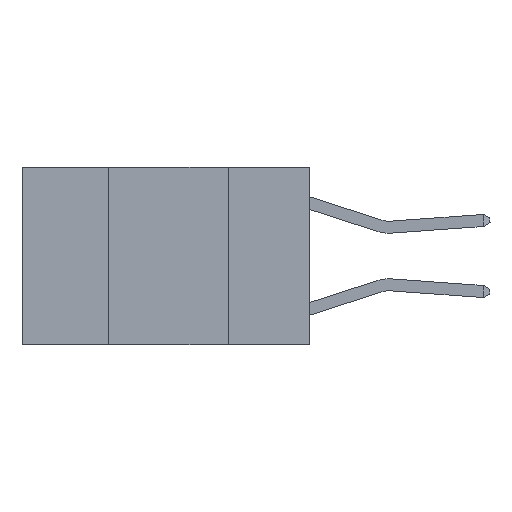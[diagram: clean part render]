
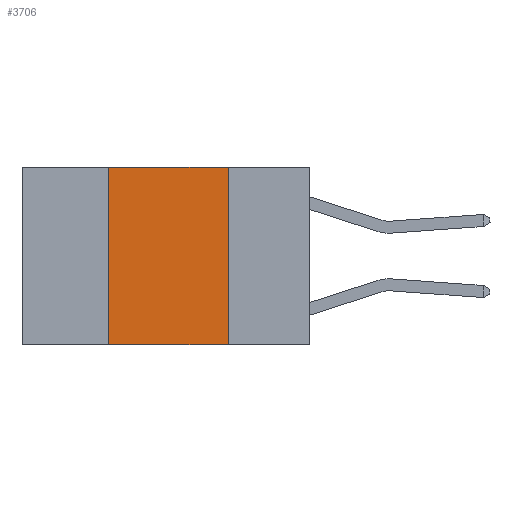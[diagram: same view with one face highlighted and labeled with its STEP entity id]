
A CAD part, left-side view. The second image highlights one B-rep face of the part: STEP entity #3706.
In plain terms, the highlighted planar face has unit normal (-1, 0, 0).
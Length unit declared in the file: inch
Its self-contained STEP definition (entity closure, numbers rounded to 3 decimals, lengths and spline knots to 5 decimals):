
#1372 = PLANE ( 'NONE',  #6216 ) ;
#1774 = EDGE_CURVE ( 'NONE', #10091, #12198, #4203, .T. ) ;
#2193 = ORIENTED_EDGE ( 'NONE', *, *, #7167, .F. ) ;
#2509 = VERTEX_POINT ( 'NONE', #12847 ) ;
#2568 = CARTESIAN_POINT ( 'NONE',  ( 0., 0.6, 0. ) ) ;
#2668 = EDGE_LOOP ( 'NONE', ( #5587, #2193, #8584, #11787 ) ) ;
#3404 = VECTOR ( 'NONE', #7515, 39.37008 ) ;
#3407 = DIRECTION ( 'NONE',  ( 0., 0., -1. ) ) ;
#3453 = EDGE_CURVE ( 'NONE', #2509, #6260, #5759, .T. ) ;
#3706 = ADVANCED_FACE ( 'NONE', ( #4728 ), #1372, .F. ) ;
#3886 = DIRECTION ( 'NONE',  ( 1., 0., 0. ) ) ;
#4203 = LINE ( 'NONE', #15080, #3404 ) ;
#4728 = FACE_OUTER_BOUND ( 'NONE', #2668, .T. ) ;
#5340 = VECTOR ( 'NONE', #3407, 39.37008 ) ;
#5442 = VECTOR ( 'NONE', #14764, 39.37008 ) ;
#5587 = ORIENTED_EDGE ( 'NONE', *, *, #3453, .F. ) ;
#5759 = LINE ( 'NONE', #13618, #5340 ) ;
#6216 = AXIS2_PLACEMENT_3D ( 'NONE', #2568, #3886, #12817 ) ;
#6260 = VERTEX_POINT ( 'NONE', #14346 ) ;
#6688 = LINE ( 'NONE', #9633, #10096 ) ;
#7045 = DIRECTION ( 'NONE',  ( 0., -1., 0. ) ) ;
#7167 = EDGE_CURVE ( 'NONE', #12198, #2509, #12240, .T. ) ;
#7515 = DIRECTION ( 'NONE',  ( 0., 0., 1. ) ) ;
#8584 = ORIENTED_EDGE ( 'NONE', *, *, #1774, .F. ) ;
#9633 = CARTESIAN_POINT ( 'NONE',  ( 0., 0.6, -0.37 ) ) ;
#10091 = VERTEX_POINT ( 'NONE', #12140 ) ;
#10096 = VECTOR ( 'NONE', #7045, 39.37008 ) ;
#11787 = ORIENTED_EDGE ( 'NONE', *, *, #14855, .T. ) ;
#12140 = CARTESIAN_POINT ( 'NONE',  ( 0., 0.42, -0.37 ) ) ;
#12198 = VERTEX_POINT ( 'NONE', #14069 ) ;
#12240 = LINE ( 'NONE', #15957, #5442 ) ;
#12817 = DIRECTION ( 'NONE',  ( 0., 0., -1. ) ) ;
#12847 = CARTESIAN_POINT ( 'NONE',  ( 0., 0.17, 0. ) ) ;
#13618 = CARTESIAN_POINT ( 'NONE',  ( 0., 0.17, 0. ) ) ;
#14069 = CARTESIAN_POINT ( 'NONE',  ( 0., 0.42, 0. ) ) ;
#14346 = CARTESIAN_POINT ( 'NONE',  ( 0., 0.17, -0.37 ) ) ;
#14764 = DIRECTION ( 'NONE',  ( 0., -1., 0. ) ) ;
#14855 = EDGE_CURVE ( 'NONE', #10091, #6260, #6688, .T. ) ;
#15080 = CARTESIAN_POINT ( 'NONE',  ( 0., 0.42, 0. ) ) ;
#15957 = CARTESIAN_POINT ( 'NONE',  ( 0., 0.6, 0. ) ) ;
